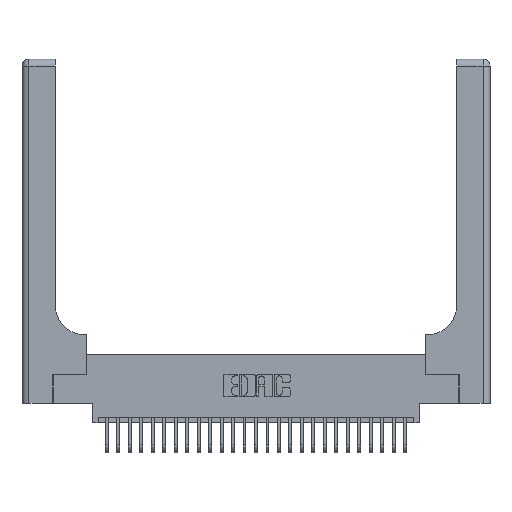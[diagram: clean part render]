
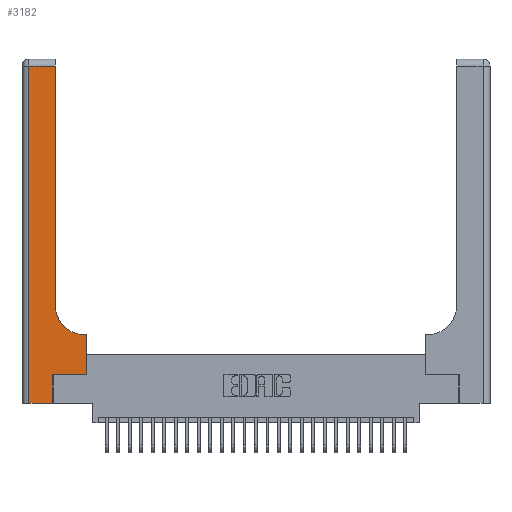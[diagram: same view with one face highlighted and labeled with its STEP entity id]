
A CAD part, top view. The second image highlights one B-rep face of the part: STEP entity #3182.
In plain terms, the highlighted planar face has unit normal (0, 0, 1).
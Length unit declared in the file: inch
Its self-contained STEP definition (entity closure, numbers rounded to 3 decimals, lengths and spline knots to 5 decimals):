
#4 = DIRECTION ( 'NONE',  ( 0., 1., 0. ) ) ;
#104 = CARTESIAN_POINT ( 'NONE',  ( 0.269, 0.25, 0.37 ) ) ;
#129 = CARTESIAN_POINT ( 'NONE',  ( 0.269, 0., 0.37 ) ) ;
#598 = VECTOR ( 'NONE', #23506, 39.37008 ) ;
#1350 = CARTESIAN_POINT ( 'NONE',  ( 0.06, 3., 0.37 ) ) ;
#1821 = CARTESIAN_POINT ( 'NONE',  ( 0.5415, 0.85, 0.37 ) ) ;
#1928 = VECTOR ( 'NONE', #4, 39.37008 ) ;
#2109 = EDGE_CURVE ( 'NONE', #8327, #21307, #5504, .T. ) ;
#2532 = CARTESIAN_POINT ( 'NONE',  ( 0.2915, 0.6, 0.37 ) ) ;
#2823 = EDGE_LOOP ( 'NONE', ( #20895, #3846, #10088, #29119, #3760, #23917, #14973, #9556, #3899 ) ) ;
#3028 = VERTEX_POINT ( 'NONE', #24243 ) ;
#3182 = ADVANCED_FACE ( 'NONE', ( #25141 ), #6481, .F. ) ;
#3699 = CARTESIAN_POINT ( 'NONE',  ( 0.06, 0., 0.37 ) ) ;
#3760 = ORIENTED_EDGE ( 'NONE', *, *, #26008, .T. ) ;
#3846 = ORIENTED_EDGE ( 'NONE', *, *, #29013, .T. ) ;
#3881 = DIRECTION ( 'NONE',  ( 1., 0., 0. ) ) ;
#3899 = ORIENTED_EDGE ( 'NONE', *, *, #14304, .T. ) ;
#4040 = VECTOR ( 'NONE', #27394, 39.37008 ) ;
#4919 = CARTESIAN_POINT ( 'NONE',  ( 0.2915, 2.94, 0.37 ) ) ;
#5405 = CARTESIAN_POINT ( 'NONE',  ( 0.269, 0.25, 0.37 ) ) ;
#5504 = LINE ( 'NONE', #8827, #23381 ) ;
#5707 = DIRECTION ( 'NONE',  ( 0., -1., 0. ) ) ;
#5901 = LINE ( 'NONE', #9459, #1928 ) ;
#5940 = EDGE_CURVE ( 'NONE', #25595, #8327, #18400, .T. ) ;
#6372 = EDGE_CURVE ( 'NONE', #24678, #26840, #29368, .T. ) ;
#6481 = PLANE ( 'NONE',  #16897 ) ;
#8327 = VERTEX_POINT ( 'NONE', #29221 ) ;
#8642 = CARTESIAN_POINT ( 'NONE',  ( 0.269, 0., 0.37 ) ) ;
#8827 = CARTESIAN_POINT ( 'NONE',  ( 0.5585, 0.25, 0.37 ) ) ;
#8855 = VERTEX_POINT ( 'NONE', #27020 ) ;
#8913 = CARTESIAN_POINT ( 'NONE',  ( 0.06, 2.94, 0.37 ) ) ;
#9027 = VERTEX_POINT ( 'NONE', #4919 ) ;
#9459 = CARTESIAN_POINT ( 'NONE',  ( 0.2915, 3., 0.37 ) ) ;
#9556 = ORIENTED_EDGE ( 'NONE', *, *, #29526, .T. ) ;
#10088 = ORIENTED_EDGE ( 'NONE', *, *, #14515, .T. ) ;
#10377 = VECTOR ( 'NONE', #20695, 39.37008 ) ;
#11090 = CARTESIAN_POINT ( 'NONE',  ( 0., 3., 0.37 ) ) ;
#11284 = DIRECTION ( 'NONE',  ( 0., 1., 0. ) ) ;
#12264 = LINE ( 'NONE', #2532, #598 ) ;
#14104 = CARTESIAN_POINT ( 'NONE',  ( 0.5585, 0.6, 0.37 ) ) ;
#14304 = EDGE_CURVE ( 'NONE', #3028, #8855, #29625, .T. ) ;
#14515 = EDGE_CURVE ( 'NONE', #18035, #24678, #15197, .T. ) ;
#14803 = VECTOR ( 'NONE', #16607, 39.37008 ) ;
#14850 = VECTOR ( 'NONE', #5707, 39.37008 ) ;
#14973 = ORIENTED_EDGE ( 'NONE', *, *, #2109, .T. ) ;
#15197 = LINE ( 'NONE', #1350, #14850 ) ;
#15661 = DIRECTION ( 'NONE',  ( -1., 0., 0. ) ) ;
#15679 = AXIS2_PLACEMENT_3D ( 'NONE', #1821, #17780, #20344 ) ;
#16607 = DIRECTION ( 'NONE',  ( -1., 0., 0. ) ) ;
#16897 = AXIS2_PLACEMENT_3D ( 'NONE', #11090, #25047, #15661 ) ;
#17780 = DIRECTION ( 'NONE',  ( 0., 0., -1. ) ) ;
#18035 = VERTEX_POINT ( 'NONE', #8913 ) ;
#18400 = LINE ( 'NONE', #5405, #25383 ) ;
#18820 = EDGE_CURVE ( 'NONE', #8855, #9027, #5901, .T. ) ;
#19145 = CARTESIAN_POINT ( 'NONE',  ( 0., 2.94, 0.37 ) ) ;
#20344 = DIRECTION ( 'NONE',  ( 1., 0., 0. ) ) ;
#20695 = DIRECTION ( 'NONE',  ( 1., 0., 0. ) ) ;
#20895 = ORIENTED_EDGE ( 'NONE', *, *, #18820, .T. ) ;
#21307 = VERTEX_POINT ( 'NONE', #14104 ) ;
#23381 = VECTOR ( 'NONE', #11284, 39.37008 ) ;
#23506 = DIRECTION ( 'NONE',  ( -1., 0., 0. ) ) ;
#23917 = ORIENTED_EDGE ( 'NONE', *, *, #5940, .T. ) ;
#24243 = CARTESIAN_POINT ( 'NONE',  ( 0.5415, 0.6, 0.37 ) ) ;
#24678 = VERTEX_POINT ( 'NONE', #3699 ) ;
#25038 = LINE ( 'NONE', #19145, #14803 ) ;
#25047 = DIRECTION ( 'NONE',  ( 0., 0., -1. ) ) ;
#25141 = FACE_OUTER_BOUND ( 'NONE', #2823, .T. ) ;
#25383 = VECTOR ( 'NONE', #3881, 39.37008 ) ;
#25595 = VERTEX_POINT ( 'NONE', #104 ) ;
#26008 = EDGE_CURVE ( 'NONE', #26840, #25595, #27370, .T. ) ;
#26840 = VERTEX_POINT ( 'NONE', #129 ) ;
#27020 = CARTESIAN_POINT ( 'NONE',  ( 0.2915, 0.85, 0.37 ) ) ;
#27370 = LINE ( 'NONE', #8642, #4040 ) ;
#27394 = DIRECTION ( 'NONE',  ( 0., 1., 0. ) ) ;
#28214 = CARTESIAN_POINT ( 'NONE',  ( 0., 0., 0.37 ) ) ;
#29013 = EDGE_CURVE ( 'NONE', #9027, #18035, #25038, .T. ) ;
#29119 = ORIENTED_EDGE ( 'NONE', *, *, #6372, .T. ) ;
#29221 = CARTESIAN_POINT ( 'NONE',  ( 0.5585, 0.25, 0.37 ) ) ;
#29368 = LINE ( 'NONE', #28214, #10377 ) ;
#29526 = EDGE_CURVE ( 'NONE', #21307, #3028, #12264, .T. ) ;
#29625 = CIRCLE ( 'NONE', #15679, 0.25 ) ;
